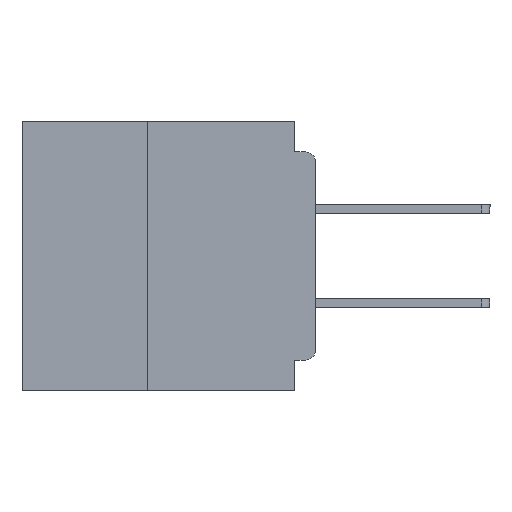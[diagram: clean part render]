
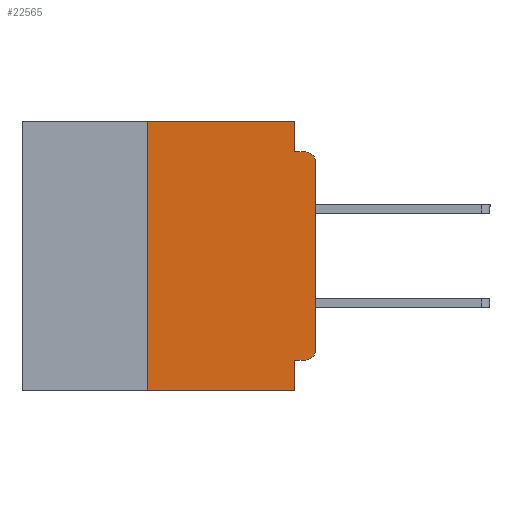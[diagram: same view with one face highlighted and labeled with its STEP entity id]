
A CAD part, left-side view. The second image highlights one B-rep face of the part: STEP entity #22565.
In plain terms, the highlighted planar face has unit normal (-1, 0, 0).
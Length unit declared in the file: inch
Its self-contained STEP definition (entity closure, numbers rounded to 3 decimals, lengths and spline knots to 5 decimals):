
#7 = LINE ( 'NONE', #16774, #25123 ) ;
#414 = VECTOR ( 'NONE', #15228, 39.37008 ) ;
#684 = FACE_OUTER_BOUND ( 'NONE', #28862, .T. ) ;
#1409 = ORIENTED_EDGE ( 'NONE', *, *, #2699, .F. ) ;
#1449 = DIRECTION ( 'NONE',  ( 0., -1., 0. ) ) ;
#1455 = CARTESIAN_POINT ( 'NONE',  ( 0., 0., -0.06 ) ) ;
#1509 = VECTOR ( 'NONE', #35147, 39.37008 ) ;
#1831 = DIRECTION ( 'NONE',  ( 0., -1., 0. ) ) ;
#2002 = EDGE_CURVE ( 'NONE', #15576, #3584, #6176, .T. ) ;
#2116 = EDGE_CURVE ( 'NONE', #23562, #37869, #7, .T. ) ;
#2699 = EDGE_CURVE ( 'NONE', #38157, #8540, #4558, .T. ) ;
#2864 = DIRECTION ( 'NONE',  ( 0., 0., -1. ) ) ;
#3099 = CARTESIAN_POINT ( 'NONE',  ( 0., 0.25, 0. ) ) ;
#3147 = CIRCLE ( 'NONE', #9431, 0.015 ) ;
#3584 = VERTEX_POINT ( 'NONE', #28052 ) ;
#3587 = LINE ( 'NONE', #41633, #1509 ) ;
#4558 = LINE ( 'NONE', #6532, #12334 ) ;
#5394 = VERTEX_POINT ( 'NONE', #37519 ) ;
#5885 = CIRCLE ( 'NONE', #40268, 0.015 ) ;
#6176 = LINE ( 'NONE', #19311, #24624 ) ;
#6532 = CARTESIAN_POINT ( 'NONE',  ( 0., 0.25, -0.4 ) ) ;
#6841 = ORIENTED_EDGE ( 'NONE', *, *, #2116, .F. ) ;
#8540 = VERTEX_POINT ( 'NONE', #3099 ) ;
#8548 = CARTESIAN_POINT ( 'NONE',  ( 0., 0.031, 0. ) ) ;
#9392 = PLANE ( 'NONE',  #16905 ) ;
#9431 = AXIS2_PLACEMENT_3D ( 'NONE', #12404, #35229, #15696 ) ;
#9935 = DIRECTION ( 'NONE',  ( -1., 0., 0. ) ) ;
#10942 = CARTESIAN_POINT ( 'NONE',  ( 0., 0.25, -0.4 ) ) ;
#12334 = VECTOR ( 'NONE', #32433, 39.37008 ) ;
#12404 = CARTESIAN_POINT ( 'NONE',  ( 0., 0.015, -0.34 ) ) ;
#12599 = CARTESIAN_POINT ( 'NONE',  ( 0., 0.437, 0. ) ) ;
#12622 = VECTOR ( 'NONE', #1449, 39.37008 ) ;
#12741 = DIRECTION ( 'NONE',  ( 0., 0., -1. ) ) ;
#13409 = CARTESIAN_POINT ( 'NONE',  ( 0., 0.015, -0.355 ) ) ;
#14733 = ORIENTED_EDGE ( 'NONE', *, *, #32940, .T. ) ;
#15228 = DIRECTION ( 'NONE',  ( 0., 0., 1. ) ) ;
#15240 = EDGE_CURVE ( 'NONE', #8540, #39628, #21238, .T. ) ;
#15576 = VERTEX_POINT ( 'NONE', #13409 ) ;
#15696 = DIRECTION ( 'NONE',  ( 0., 0., -1. ) ) ;
#16374 = VECTOR ( 'NONE', #2864, 39.37008 ) ;
#16774 = CARTESIAN_POINT ( 'NONE',  ( 0., 0., -0.045 ) ) ;
#16905 = AXIS2_PLACEMENT_3D ( 'NONE', #12599, #32274, #12741 ) ;
#17357 = VERTEX_POINT ( 'NONE', #41848 ) ;
#17381 = LINE ( 'NONE', #35483, #16374 ) ;
#17833 = LINE ( 'NONE', #18177, #414 ) ;
#18177 = CARTESIAN_POINT ( 'NONE',  ( 0., 0., 0. ) ) ;
#19311 = CARTESIAN_POINT ( 'NONE',  ( 0., 0., -0.355 ) ) ;
#19482 = ORIENTED_EDGE ( 'NONE', *, *, #20823, .F. ) ;
#20019 = DIRECTION ( 'NONE',  ( 0., -1., 0. ) ) ;
#20304 = VECTOR ( 'NONE', #1831, 39.37008 ) ;
#20823 = EDGE_CURVE ( 'NONE', #39628, #23562, #17381, .T. ) ;
#21238 = LINE ( 'NONE', #24362, #12622 ) ;
#21324 = LINE ( 'NONE', #40985, #20304 ) ;
#22565 = ADVANCED_FACE ( 'NONE', ( #684 ), #9392, .F. ) ;
#23405 = ORIENTED_EDGE ( 'NONE', *, *, #24328, .F. ) ;
#23562 = VERTEX_POINT ( 'NONE', #40998 ) ;
#24328 = EDGE_CURVE ( 'NONE', #3584, #5394, #3587, .T. ) ;
#24362 = CARTESIAN_POINT ( 'NONE',  ( 0., 0.437, 0. ) ) ;
#24624 = VECTOR ( 'NONE', #35624, 39.37008 ) ;
#25123 = VECTOR ( 'NONE', #20019, 39.37008 ) ;
#28052 = CARTESIAN_POINT ( 'NONE',  ( 0., 0.031, -0.355 ) ) ;
#28862 = EDGE_LOOP ( 'NONE', ( #14733, #39846, #6841, #19482, #30849, #1409, #41158, #23405, #29985, #30787 ) ) ;
#29512 = CARTESIAN_POINT ( 'NONE',  ( 0., 0.015, -0.06 ) ) ;
#29985 = ORIENTED_EDGE ( 'NONE', *, *, #2002, .F. ) ;
#30228 = EDGE_CURVE ( 'NONE', #15576, #17357, #3147, .T. ) ;
#30787 = ORIENTED_EDGE ( 'NONE', *, *, #30228, .T. ) ;
#30849 = ORIENTED_EDGE ( 'NONE', *, *, #15240, .F. ) ;
#32274 = DIRECTION ( 'NONE',  ( 1., 0., 0. ) ) ;
#32433 = DIRECTION ( 'NONE',  ( 0., 0., 1. ) ) ;
#32802 = DIRECTION ( 'NONE',  ( 0., 0., -1. ) ) ;
#32940 = EDGE_CURVE ( 'NONE', #17357, #40258, #17833, .T. ) ;
#35057 = EDGE_CURVE ( 'NONE', #38157, #5394, #21324, .T. ) ;
#35147 = DIRECTION ( 'NONE',  ( 0., 0., -1. ) ) ;
#35229 = DIRECTION ( 'NONE',  ( -1., 0., 0. ) ) ;
#35483 = CARTESIAN_POINT ( 'NONE',  ( 0., 0.031, 0. ) ) ;
#35624 = DIRECTION ( 'NONE',  ( 0., 1., 0. ) ) ;
#36523 = EDGE_CURVE ( 'NONE', #40258, #37869, #5885, .T. ) ;
#37519 = CARTESIAN_POINT ( 'NONE',  ( 0., 0.031, -0.4 ) ) ;
#37869 = VERTEX_POINT ( 'NONE', #41194 ) ;
#38157 = VERTEX_POINT ( 'NONE', #10942 ) ;
#39628 = VERTEX_POINT ( 'NONE', #8548 ) ;
#39846 = ORIENTED_EDGE ( 'NONE', *, *, #36523, .T. ) ;
#40258 = VERTEX_POINT ( 'NONE', #1455 ) ;
#40268 = AXIS2_PLACEMENT_3D ( 'NONE', #29512, #9935, #32802 ) ;
#40985 = CARTESIAN_POINT ( 'NONE',  ( 0., 0.437, -0.4 ) ) ;
#40998 = CARTESIAN_POINT ( 'NONE',  ( 0., 0.031, -0.045 ) ) ;
#41158 = ORIENTED_EDGE ( 'NONE', *, *, #35057, .T. ) ;
#41194 = CARTESIAN_POINT ( 'NONE',  ( 0., 0.015, -0.045 ) ) ;
#41633 = CARTESIAN_POINT ( 'NONE',  ( 0., 0.031, -0.4 ) ) ;
#41848 = CARTESIAN_POINT ( 'NONE',  ( 0., 0., -0.34 ) ) ;
